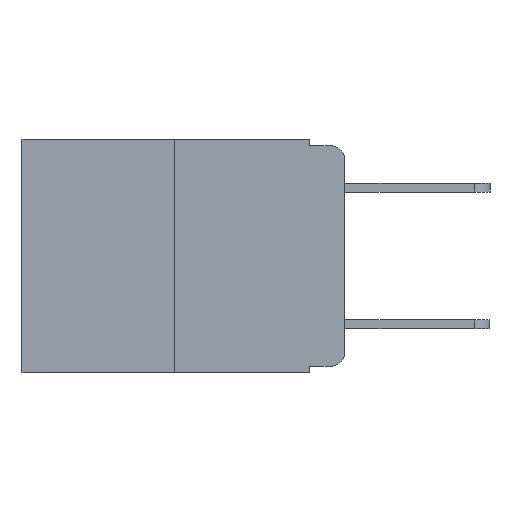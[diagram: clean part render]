
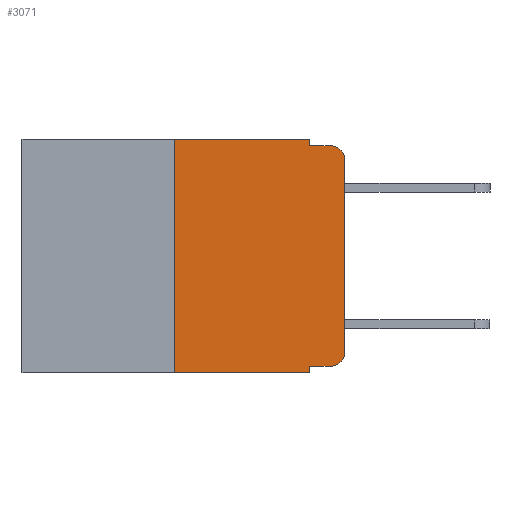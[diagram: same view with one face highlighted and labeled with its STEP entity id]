
A CAD part, left-side view. The second image highlights one B-rep face of the part: STEP entity #3071.
In plain terms, the highlighted planar face has unit normal (-1, 0, 0).
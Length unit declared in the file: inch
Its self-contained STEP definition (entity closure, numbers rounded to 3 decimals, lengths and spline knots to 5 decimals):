
#139 = VERTEX_POINT ( 'NONE', #9236 ) ;
#173 = ORIENTED_EDGE ( 'NONE', *, *, #6629, .T. ) ;
#233 = CARTESIAN_POINT ( 'NONE',  ( 0., 0.473, -0.343 ) ) ;
#444 = CARTESIAN_POINT ( 'NONE',  ( 0., 0.473, 0. ) ) ;
#732 = VERTEX_POINT ( 'NONE', #3348 ) ;
#836 = DIRECTION ( 'NONE',  ( 0., -1., 0. ) ) ;
#931 = CARTESIAN_POINT ( 'NONE',  ( 0., 0.25, 0. ) ) ;
#937 = VECTOR ( 'NONE', #6281, 39.37008 ) ;
#1523 = DIRECTION ( 'NONE',  ( 0., -1., 0. ) ) ;
#1757 = VERTEX_POINT ( 'NONE', #3747 ) ;
#1779 = VERTEX_POINT ( 'NONE', #9062 ) ;
#1852 = CARTESIAN_POINT ( 'NONE',  ( 0., 0.051, -0.01 ) ) ;
#1884 = LINE ( 'NONE', #233, #4549 ) ;
#2191 = VECTOR ( 'NONE', #9050, 39.37008 ) ;
#2295 = DIRECTION ( 'NONE',  ( 1., 0., 0. ) ) ;
#2307 = ORIENTED_EDGE ( 'NONE', *, *, #7065, .F. ) ;
#2471 = EDGE_LOOP ( 'NONE', ( #4362, #8404, #2307, #8625, #10518, #6969, #173, #2864, #5145, #7194 ) ) ;
#2583 = VERTEX_POINT ( 'NONE', #3157 ) ;
#2864 = ORIENTED_EDGE ( 'NONE', *, *, #7207, .F. ) ;
#2901 = CIRCLE ( 'NONE', #7952, 0.02 ) ;
#3071 = ADVANCED_FACE ( 'NONE', ( #7523 ), #6474, .F. ) ;
#3157 = CARTESIAN_POINT ( 'NONE',  ( 0., 0.25, -0.343 ) ) ;
#3174 = VECTOR ( 'NONE', #7057, 39.37008 ) ;
#3348 = CARTESIAN_POINT ( 'NONE',  ( 0., 0.02, -0.01 ) ) ;
#3454 = LINE ( 'NONE', #9166, #3174 ) ;
#3615 = CARTESIAN_POINT ( 'NONE',  ( 0., 0.051, 0. ) ) ;
#3747 = CARTESIAN_POINT ( 'NONE',  ( 0., 0., -0.03 ) ) ;
#4076 = DIRECTION ( 'NONE',  ( 0., -1., 0. ) ) ;
#4261 = LINE ( 'NONE', #931, #8090 ) ;
#4362 = ORIENTED_EDGE ( 'NONE', *, *, #7049, .T. ) ;
#4515 = CARTESIAN_POINT ( 'NONE',  ( 0., 0., 0. ) ) ;
#4549 = VECTOR ( 'NONE', #4076, 39.37008 ) ;
#4556 = LINE ( 'NONE', #444, #8104 ) ;
#4782 = DIRECTION ( 'NONE',  ( -1., 0., 0. ) ) ;
#4811 = CIRCLE ( 'NONE', #4927, 0.02 ) ;
#4927 = AXIS2_PLACEMENT_3D ( 'NONE', #9785, #5380, #10466 ) ;
#5145 = ORIENTED_EDGE ( 'NONE', *, *, #7224, .T. ) ;
#5380 = DIRECTION ( 'NONE',  ( -1., 0., 0. ) ) ;
#5419 = DIRECTION ( 'NONE',  ( 0., 0., 1. ) ) ;
#5896 = VERTEX_POINT ( 'NONE', #10118 ) ;
#6024 = EDGE_CURVE ( 'NONE', #139, #10305, #4556, .T. ) ;
#6174 = CARTESIAN_POINT ( 'NONE',  ( 0., 0.051, 0. ) ) ;
#6281 = DIRECTION ( 'NONE',  ( 0., 0., -1. ) ) ;
#6283 = CARTESIAN_POINT ( 'NONE',  ( 0., 0., -0.313 ) ) ;
#6363 = AXIS2_PLACEMENT_3D ( 'NONE', #7213, #2295, #7923 ) ;
#6474 = PLANE ( 'NONE',  #6363 ) ;
#6629 = EDGE_CURVE ( 'NONE', #2583, #5896, #1884, .T. ) ;
#6648 = VECTOR ( 'NONE', #836, 39.37008 ) ;
#6891 = VECTOR ( 'NONE', #10434, 39.37008 ) ;
#6969 = ORIENTED_EDGE ( 'NONE', *, *, #7104, .F. ) ;
#7049 = EDGE_CURVE ( 'NONE', #10616, #1757, #9010, .T. ) ;
#7057 = DIRECTION ( 'NONE',  ( 0., -1., 0. ) ) ;
#7062 = EDGE_CURVE ( 'NONE', #1757, #732, #4811, .T. ) ;
#7065 = EDGE_CURVE ( 'NONE', #9382, #732, #8552, .T. ) ;
#7068 = CARTESIAN_POINT ( 'NONE',  ( 0., 0.02, -0.333 ) ) ;
#7076 = EDGE_CURVE ( 'NONE', #10305, #9382, #8780, .T. ) ;
#7104 = EDGE_CURVE ( 'NONE', #2583, #139, #4261, .T. ) ;
#7194 = ORIENTED_EDGE ( 'NONE', *, *, #7255, .T. ) ;
#7207 = EDGE_CURVE ( 'NONE', #1779, #5896, #7680, .T. ) ;
#7213 = CARTESIAN_POINT ( 'NONE',  ( 0., 0.473, 0. ) ) ;
#7224 = EDGE_CURVE ( 'NONE', #1779, #9482, #3454, .T. ) ;
#7255 = EDGE_CURVE ( 'NONE', #9482, #10616, #2901, .T. ) ;
#7523 = FACE_OUTER_BOUND ( 'NONE', #2471, .T. ) ;
#7637 = CARTESIAN_POINT ( 'NONE',  ( 0., 0.051, -0.01 ) ) ;
#7680 = LINE ( 'NONE', #8412, #937 ) ;
#7923 = DIRECTION ( 'NONE',  ( 0., 0., -1. ) ) ;
#7952 = AXIS2_PLACEMENT_3D ( 'NONE', #9218, #4782, #9960 ) ;
#8090 = VECTOR ( 'NONE', #5419, 39.37008 ) ;
#8104 = VECTOR ( 'NONE', #1523, 39.37008 ) ;
#8404 = ORIENTED_EDGE ( 'NONE', *, *, #7062, .T. ) ;
#8412 = CARTESIAN_POINT ( 'NONE',  ( 0., 0.051, 0. ) ) ;
#8552 = LINE ( 'NONE', #7637, #6648 ) ;
#8625 = ORIENTED_EDGE ( 'NONE', *, *, #7076, .F. ) ;
#8780 = LINE ( 'NONE', #6174, #2191 ) ;
#9010 = LINE ( 'NONE', #4515, #6891 ) ;
#9050 = DIRECTION ( 'NONE',  ( 0., 0., -1. ) ) ;
#9062 = CARTESIAN_POINT ( 'NONE',  ( 0., 0.051, -0.333 ) ) ;
#9166 = CARTESIAN_POINT ( 'NONE',  ( 0., 0.051, -0.333 ) ) ;
#9218 = CARTESIAN_POINT ( 'NONE',  ( 0., 0.02, -0.313 ) ) ;
#9236 = CARTESIAN_POINT ( 'NONE',  ( 0., 0.25, 0. ) ) ;
#9382 = VERTEX_POINT ( 'NONE', #1852 ) ;
#9482 = VERTEX_POINT ( 'NONE', #7068 ) ;
#9785 = CARTESIAN_POINT ( 'NONE',  ( 0., 0.02, -0.03 ) ) ;
#9960 = DIRECTION ( 'NONE',  ( 0., 0., -1. ) ) ;
#10118 = CARTESIAN_POINT ( 'NONE',  ( 0., 0.051, -0.343 ) ) ;
#10305 = VERTEX_POINT ( 'NONE', #3615 ) ;
#10434 = DIRECTION ( 'NONE',  ( 0., 0., 1. ) ) ;
#10466 = DIRECTION ( 'NONE',  ( 0., 0., -1. ) ) ;
#10518 = ORIENTED_EDGE ( 'NONE', *, *, #6024, .F. ) ;
#10616 = VERTEX_POINT ( 'NONE', #6283 ) ;
